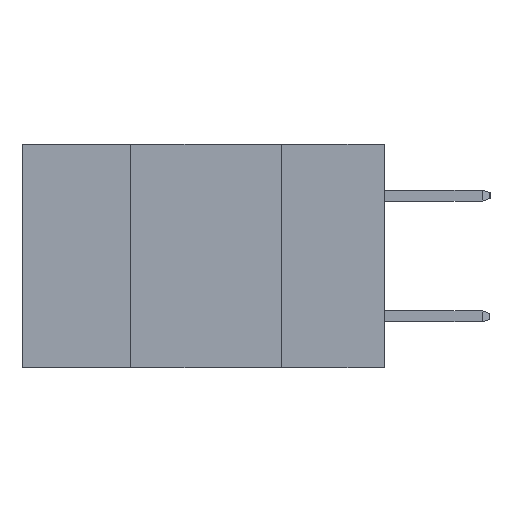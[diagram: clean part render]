
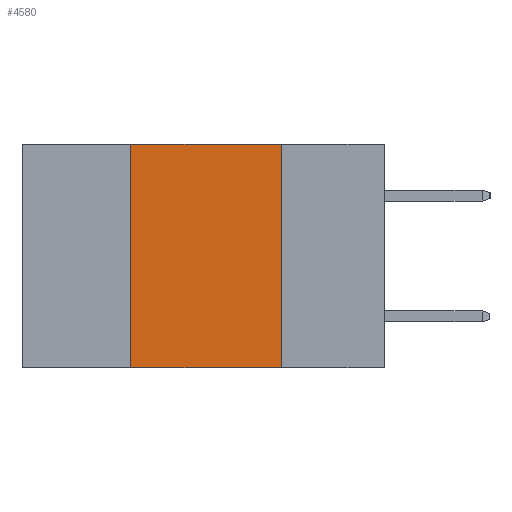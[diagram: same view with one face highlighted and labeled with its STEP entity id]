
A CAD part, left-side view. The second image highlights one B-rep face of the part: STEP entity #4580.
In plain terms, the highlighted planar face has unit normal (-1, 0, 0).
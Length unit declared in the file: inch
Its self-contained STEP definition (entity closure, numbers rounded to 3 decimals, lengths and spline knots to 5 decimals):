
#422 = ORIENTED_EDGE ( 'NONE', *, *, #1983, .T. ) ;
#659 = EDGE_LOOP ( 'NONE', ( #11549, #947, #759, #422 ) ) ;
#759 = ORIENTED_EDGE ( 'NONE', *, *, #8643, .F. ) ;
#947 = ORIENTED_EDGE ( 'NONE', *, *, #11102, .F. ) ;
#1285 = VERTEX_POINT ( 'NONE', #7454 ) ;
#1935 = DIRECTION ( 'NONE',  ( 0., -1., 0. ) ) ;
#1983 = EDGE_CURVE ( 'NONE', #2970, #9514, #8719, .T. ) ;
#2157 = DIRECTION ( 'NONE',  ( 0., 0., -1. ) ) ;
#2272 = VERTEX_POINT ( 'NONE', #2754 ) ;
#2359 = LINE ( 'NONE', #6718, #7160 ) ;
#2543 = AXIS2_PLACEMENT_3D ( 'NONE', #3073, #6671, #3127 ) ;
#2754 = CARTESIAN_POINT ( 'NONE',  ( 0., 0.17, 0. ) ) ;
#2887 = VECTOR ( 'NONE', #9544, 39.37008 ) ;
#2970 = VERTEX_POINT ( 'NONE', #8379 ) ;
#3073 = CARTESIAN_POINT ( 'NONE',  ( 0., 0.6, 0. ) ) ;
#3127 = DIRECTION ( 'NONE',  ( 0., 0., -1. ) ) ;
#3393 = FACE_OUTER_BOUND ( 'NONE', #659, .T. ) ;
#3995 = DIRECTION ( 'NONE',  ( 0., -1., 0. ) ) ;
#4089 = CARTESIAN_POINT ( 'NONE',  ( 0., 0.6, -0.37 ) ) ;
#4490 = CARTESIAN_POINT ( 'NONE',  ( 0., 0.17, 0. ) ) ;
#4566 = LINE ( 'NONE', #4490, #7111 ) ;
#4580 = ADVANCED_FACE ( 'NONE', ( #3393 ), #6634, .F. ) ;
#4887 = EDGE_CURVE ( 'NONE', #2272, #9514, #4566, .T. ) ;
#6253 = VECTOR ( 'NONE', #3995, 39.37008 ) ;
#6634 = PLANE ( 'NONE',  #2543 ) ;
#6671 = DIRECTION ( 'NONE',  ( 1., 0., 0. ) ) ;
#6718 = CARTESIAN_POINT ( 'NONE',  ( 0., 0.6, 0. ) ) ;
#7111 = VECTOR ( 'NONE', #2157, 39.37008 ) ;
#7160 = VECTOR ( 'NONE', #1935, 39.37008 ) ;
#7304 = CARTESIAN_POINT ( 'NONE',  ( 0., 0.42, 0. ) ) ;
#7454 = CARTESIAN_POINT ( 'NONE',  ( 0., 0.42, 0. ) ) ;
#7909 = LINE ( 'NONE', #7304, #2887 ) ;
#8379 = CARTESIAN_POINT ( 'NONE',  ( 0., 0.42, -0.37 ) ) ;
#8643 = EDGE_CURVE ( 'NONE', #2970, #1285, #7909, .T. ) ;
#8719 = LINE ( 'NONE', #4089, #6253 ) ;
#9514 = VERTEX_POINT ( 'NONE', #10267 ) ;
#9544 = DIRECTION ( 'NONE',  ( 0., 0., 1. ) ) ;
#10267 = CARTESIAN_POINT ( 'NONE',  ( 0., 0.17, -0.37 ) ) ;
#11102 = EDGE_CURVE ( 'NONE', #1285, #2272, #2359, .T. ) ;
#11549 = ORIENTED_EDGE ( 'NONE', *, *, #4887, .F. ) ;
